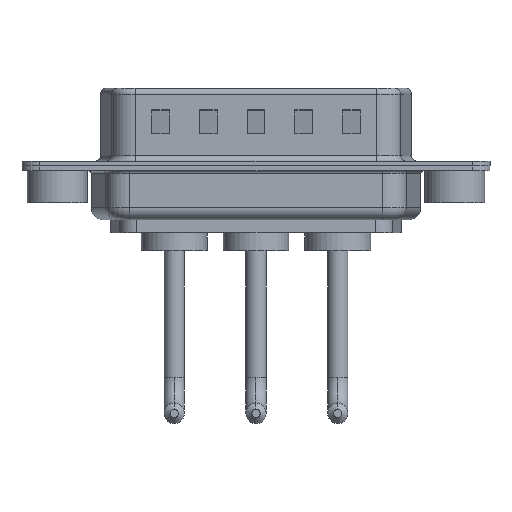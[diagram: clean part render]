
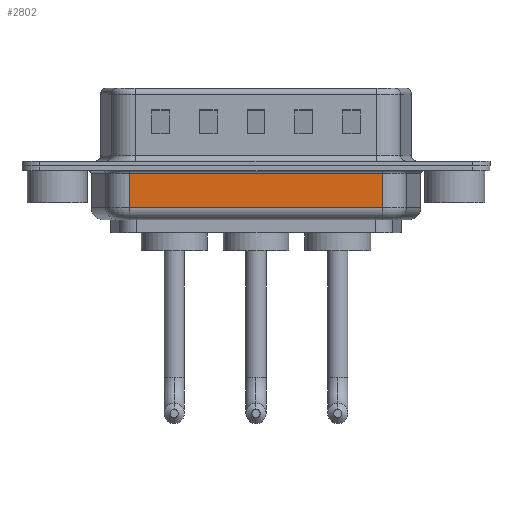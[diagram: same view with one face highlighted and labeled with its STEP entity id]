
A CAD part, front view. The second image highlights one B-rep face of the part: STEP entity #2802.
In plain terms, the highlighted planar face has unit normal (0, -1, 0).
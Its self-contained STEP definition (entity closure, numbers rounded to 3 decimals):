
#108 = ORIENTED_EDGE ( 'NONE', *, *, #15170, .F. ) ;
#492 = PLANE ( 'NONE',  #1803 ) ;
#918 = CARTESIAN_POINT ( 'NONE',  ( 6.031, -5.35, -0.65 ) ) ;
#1629 = CARTESIAN_POINT ( 'NONE',  ( 6.031, -5.35, -3.5 ) ) ;
#1803 = AXIS2_PLACEMENT_3D ( 'NONE', #4231, #12654, #5346 ) ;
#1844 = DIRECTION ( 'NONE',  ( 0., 0., 1. ) ) ;
#2802 = ADVANCED_FACE ( 'NONE', ( #12411 ), #492, .F. ) ;
#4021 = EDGE_LOOP ( 'NONE', ( #108, #8547, #10083, #7603 ) ) ;
#4070 = CARTESIAN_POINT ( 'NONE',  ( 27.269, -5.35, -4.5 ) ) ;
#4231 = CARTESIAN_POINT ( 'NONE',  ( 6.031, -5.35, -4.5 ) ) ;
#4539 = VECTOR ( 'NONE', #7987, 1000. ) ;
#4993 = VERTEX_POINT ( 'NONE', #9412 ) ;
#5014 = VERTEX_POINT ( 'NONE', #918 ) ;
#5346 = DIRECTION ( 'NONE',  ( 0., 0., 1. ) ) ;
#5917 = LINE ( 'NONE', #15709, #13404 ) ;
#5949 = LINE ( 'NONE', #14671, #4539 ) ;
#6543 = LINE ( 'NONE', #1629, #10358 ) ;
#7398 = VERTEX_POINT ( 'NONE', #13232 ) ;
#7603 = ORIENTED_EDGE ( 'NONE', *, *, #12767, .T. ) ;
#7987 = DIRECTION ( 'NONE',  ( -1., 0., 0. ) ) ;
#8081 = CARTESIAN_POINT ( 'NONE',  ( 27.269, -5.35, -3.5 ) ) ;
#8547 = ORIENTED_EDGE ( 'NONE', *, *, #12833, .T. ) ;
#9412 = CARTESIAN_POINT ( 'NONE',  ( 27.269, -5.35, -0.65 ) ) ;
#9532 = VERTEX_POINT ( 'NONE', #8081 ) ;
#10078 = LINE ( 'NONE', #4070, #15162 ) ;
#10083 = ORIENTED_EDGE ( 'NONE', *, *, #10798, .T. ) ;
#10358 = VECTOR ( 'NONE', #13630, 1000. ) ;
#10798 = EDGE_CURVE ( 'NONE', #9532, #4993, #10078, .T. ) ;
#12411 = FACE_OUTER_BOUND ( 'NONE', #4021, .T. ) ;
#12654 = DIRECTION ( 'NONE',  ( 0., 1., 0. ) ) ;
#12767 = EDGE_CURVE ( 'NONE', #4993, #5014, #5949, .T. ) ;
#12833 = EDGE_CURVE ( 'NONE', #7398, #9532, #6543, .T. ) ;
#12912 = DIRECTION ( 'NONE',  ( 0., 0., 1. ) ) ;
#13232 = CARTESIAN_POINT ( 'NONE',  ( 6.031, -5.35, -3.5 ) ) ;
#13404 = VECTOR ( 'NONE', #12912, 1000. ) ;
#13630 = DIRECTION ( 'NONE',  ( 1., 0., 0. ) ) ;
#14671 = CARTESIAN_POINT ( 'NONE',  ( 6.031, -5.35, -0.65 ) ) ;
#15162 = VECTOR ( 'NONE', #1844, 1000. ) ;
#15170 = EDGE_CURVE ( 'NONE', #7398, #5014, #5917, .T. ) ;
#15709 = CARTESIAN_POINT ( 'NONE',  ( 6.031, -5.35, -4.5 ) ) ;
